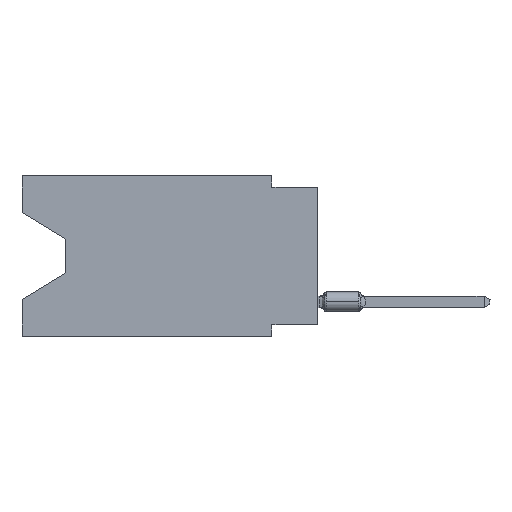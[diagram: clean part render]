
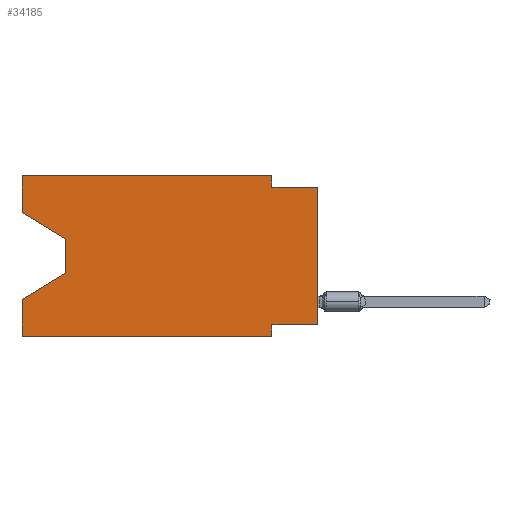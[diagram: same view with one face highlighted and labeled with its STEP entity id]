
A CAD part, left-side view. The second image highlights one B-rep face of the part: STEP entity #34185.
In plain terms, the highlighted planar face has unit normal (-1, 0, 0).
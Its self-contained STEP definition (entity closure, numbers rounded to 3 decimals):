
#1242 = CARTESIAN_POINT ( 'NONE',  ( 0., 16.383, 0. ) ) ;
#1675 = ORIENTED_EDGE ( 'NONE', *, *, #33287, .F. ) ;
#1907 = CARTESIAN_POINT ( 'NONE',  ( 0., 2.54, -8.89 ) ) ;
#2289 = ORIENTED_EDGE ( 'NONE', *, *, #17502, .F. ) ;
#2420 = LINE ( 'NONE', #5813, #15300 ) ;
#2835 = CARTESIAN_POINT ( 'NONE',  ( 0., 16.383, 0. ) ) ;
#3086 = EDGE_LOOP ( 'NONE', ( #34770, #8997, #15921, #13571, #7691, #23498, #13279, #32342, #9979, #1675, #39136, #2289 ) ) ;
#3212 = EDGE_CURVE ( 'NONE', #23391, #20350, #5331, .T. ) ;
#3217 = CARTESIAN_POINT ( 'NONE',  ( 0., 13.97, -3.505 ) ) ;
#4124 = CARTESIAN_POINT ( 'NONE',  ( 0., 2.54, 0. ) ) ;
#4370 = DIRECTION ( 'NONE',  ( 0., 0., -1. ) ) ;
#4693 = CARTESIAN_POINT ( 'NONE',  ( 0., 16.383, -8.89 ) ) ;
#4955 = DIRECTION ( 'NONE',  ( 0., 0., 1. ) ) ;
#5331 = LINE ( 'NONE', #4693, #24437 ) ;
#5487 = LINE ( 'NONE', #6119, #7157 ) ;
#5560 = LINE ( 'NONE', #18561, #35622 ) ;
#5677 = EDGE_CURVE ( 'NONE', #8256, #6456, #19574, .T. ) ;
#5813 = CARTESIAN_POINT ( 'NONE',  ( 0., 16.383, 0. ) ) ;
#5823 = LINE ( 'NONE', #2835, #31055 ) ;
#5913 = CARTESIAN_POINT ( 'NONE',  ( 0., 2.54, -0.635 ) ) ;
#6119 = CARTESIAN_POINT ( 'NONE',  ( 0., 16.383, -2.038 ) ) ;
#6456 = VERTEX_POINT ( 'NONE', #17459 ) ;
#7157 = VECTOR ( 'NONE', #38086, 1000. ) ;
#7691 = ORIENTED_EDGE ( 'NONE', *, *, #3212, .T. ) ;
#7954 = DIRECTION ( 'NONE',  ( 0., -1., 0. ) ) ;
#8256 = VERTEX_POINT ( 'NONE', #3217 ) ;
#8997 = ORIENTED_EDGE ( 'NONE', *, *, #5677, .T. ) ;
#9979 = ORIENTED_EDGE ( 'NONE', *, *, #41585, .F. ) ;
#10156 = CARTESIAN_POINT ( 'NONE',  ( 0., 0., 0. ) ) ;
#10371 = EDGE_CURVE ( 'NONE', #37325, #8256, #5487, .T. ) ;
#10480 = VERTEX_POINT ( 'NONE', #5913 ) ;
#11137 = CARTESIAN_POINT ( 'NONE',  ( 0., 0., -0.635 ) ) ;
#12231 = VECTOR ( 'NONE', #4370, 1000. ) ;
#12461 = VERTEX_POINT ( 'NONE', #1242 ) ;
#13279 = ORIENTED_EDGE ( 'NONE', *, *, #27302, .F. ) ;
#13571 = ORIENTED_EDGE ( 'NONE', *, *, #16327, .F. ) ;
#13954 = LINE ( 'NONE', #10156, #41079 ) ;
#14290 = VERTEX_POINT ( 'NONE', #19835 ) ;
#14602 = VECTOR ( 'NONE', #27462, 1000. ) ;
#14997 = CARTESIAN_POINT ( 'NONE',  ( 0., 0., -0.635 ) ) ;
#15300 = VECTOR ( 'NONE', #4955, 1000. ) ;
#15361 = CARTESIAN_POINT ( 'NONE',  ( 0., 2.54, -8.255 ) ) ;
#15867 = VECTOR ( 'NONE', #7954, 1000. ) ;
#15921 = ORIENTED_EDGE ( 'NONE', *, *, #22886, .T. ) ;
#15942 = DIRECTION ( 'NONE',  ( 0., 0., -1. ) ) ;
#16327 = EDGE_CURVE ( 'NONE', #23391, #20852, #2420, .T. ) ;
#17405 = CARTESIAN_POINT ( 'NONE',  ( 0., 13.97, -5.385 ) ) ;
#17459 = CARTESIAN_POINT ( 'NONE',  ( 0., 13.97, -5.385 ) ) ;
#17502 = EDGE_CURVE ( 'NONE', #37325, #12461, #5823, .T. ) ;
#17803 = DIRECTION ( 'NONE',  ( 0., 0.855, -0.519 ) ) ;
#18561 = CARTESIAN_POINT ( 'NONE',  ( 0., 16.383, 0. ) ) ;
#18918 = VECTOR ( 'NONE', #19966, 1000. ) ;
#19310 = DIRECTION ( 'NONE',  ( 1., 0., 0. ) ) ;
#19574 = LINE ( 'NONE', #32132, #38992 ) ;
#19835 = CARTESIAN_POINT ( 'NONE',  ( 0., 0., -8.255 ) ) ;
#19966 = DIRECTION ( 'NONE',  ( 0., 1., 0. ) ) ;
#20350 = VERTEX_POINT ( 'NONE', #37903 ) ;
#20592 = LINE ( 'NONE', #17405, #31902 ) ;
#20852 = VERTEX_POINT ( 'NONE', #22245 ) ;
#21252 = EDGE_CURVE ( 'NONE', #12461, #32932, #5560, .T. ) ;
#21498 = CARTESIAN_POINT ( 'NONE',  ( 0., 16.383, -2.038 ) ) ;
#21780 = AXIS2_PLACEMENT_3D ( 'NONE', #29329, #19310, #22504 ) ;
#22161 = VERTEX_POINT ( 'NONE', #15361 ) ;
#22245 = CARTESIAN_POINT ( 'NONE',  ( 0., 16.383, -6.852 ) ) ;
#22504 = DIRECTION ( 'NONE',  ( 0., 0., -1. ) ) ;
#22587 = EDGE_CURVE ( 'NONE', #22161, #20350, #28095, .T. ) ;
#22886 = EDGE_CURVE ( 'NONE', #6456, #20852, #20592, .T. ) ;
#23391 = VERTEX_POINT ( 'NONE', #24786 ) ;
#23498 = ORIENTED_EDGE ( 'NONE', *, *, #22587, .F. ) ;
#24437 = VECTOR ( 'NONE', #34513, 1000. ) ;
#24786 = CARTESIAN_POINT ( 'NONE',  ( 0., 16.383, -8.89 ) ) ;
#26021 = DIRECTION ( 'NONE',  ( 0., -1., 0. ) ) ;
#27170 = LINE ( 'NONE', #30369, #12231 ) ;
#27302 = EDGE_CURVE ( 'NONE', #14290, #22161, #36160, .T. ) ;
#27462 = DIRECTION ( 'NONE',  ( 0., 0., -1. ) ) ;
#28095 = LINE ( 'NONE', #1907, #14602 ) ;
#29329 = CARTESIAN_POINT ( 'NONE',  ( 0., 16.383, 0. ) ) ;
#30369 = CARTESIAN_POINT ( 'NONE',  ( 0., 2.54, 0. ) ) ;
#31055 = VECTOR ( 'NONE', #37560, 1000. ) ;
#31469 = VERTEX_POINT ( 'NONE', #14997 ) ;
#31902 = VECTOR ( 'NONE', #17803, 1000. ) ;
#32132 = CARTESIAN_POINT ( 'NONE',  ( 0., 13.97, -3.505 ) ) ;
#32342 = ORIENTED_EDGE ( 'NONE', *, *, #41089, .T. ) ;
#32932 = VERTEX_POINT ( 'NONE', #4124 ) ;
#33150 = DIRECTION ( 'NONE',  ( 0., 0., 1. ) ) ;
#33287 = EDGE_CURVE ( 'NONE', #32932, #10480, #27170, .T. ) ;
#34185 = ADVANCED_FACE ( 'NONE', ( #41901 ), #35502, .F. ) ;
#34513 = DIRECTION ( 'NONE',  ( 0., -1., 0. ) ) ;
#34770 = ORIENTED_EDGE ( 'NONE', *, *, #10371, .T. ) ;
#35502 = PLANE ( 'NONE',  #21780 ) ;
#35622 = VECTOR ( 'NONE', #26021, 1000. ) ;
#36160 = LINE ( 'NONE', #39994, #18918 ) ;
#37325 = VERTEX_POINT ( 'NONE', #21498 ) ;
#37560 = DIRECTION ( 'NONE',  ( 0., 0., 1. ) ) ;
#37903 = CARTESIAN_POINT ( 'NONE',  ( 0., 2.54, -8.89 ) ) ;
#38086 = DIRECTION ( 'NONE',  ( 0., -0.855, -0.519 ) ) ;
#38992 = VECTOR ( 'NONE', #15942, 1000. ) ;
#39136 = ORIENTED_EDGE ( 'NONE', *, *, #21252, .F. ) ;
#39994 = CARTESIAN_POINT ( 'NONE',  ( 0., 0., -8.255 ) ) ;
#40317 = LINE ( 'NONE', #11137, #15867 ) ;
#41079 = VECTOR ( 'NONE', #33150, 1000. ) ;
#41089 = EDGE_CURVE ( 'NONE', #14290, #31469, #13954, .T. ) ;
#41585 = EDGE_CURVE ( 'NONE', #10480, #31469, #40317, .T. ) ;
#41901 = FACE_OUTER_BOUND ( 'NONE', #3086, .T. ) ;
